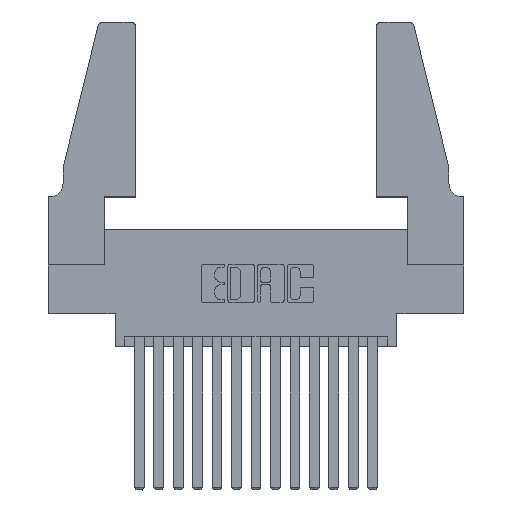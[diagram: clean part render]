
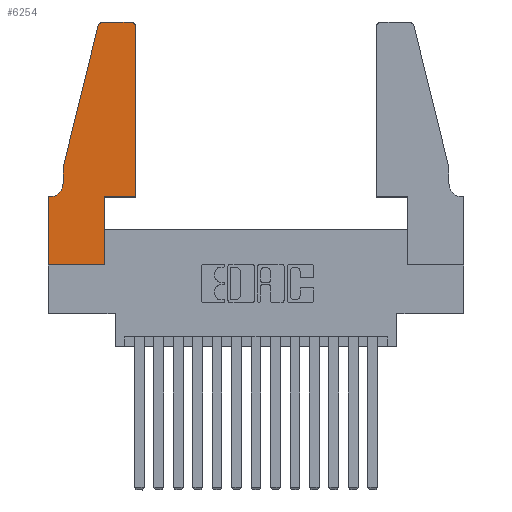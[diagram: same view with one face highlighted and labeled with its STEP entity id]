
A CAD part, top view. The second image highlights one B-rep face of the part: STEP entity #6254.
In plain terms, the highlighted planar face has unit normal (0, 0, 1).
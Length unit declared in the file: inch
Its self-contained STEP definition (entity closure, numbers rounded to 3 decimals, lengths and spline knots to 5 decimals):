
#33 = VERTEX_POINT ( 'NONE', #5022 ) ;
#185 = VECTOR ( 'NONE', #2375, 39.37008 ) ;
#260 = CARTESIAN_POINT ( 'NONE',  ( 0.2605, 1.25, 0.37 ) ) ;
#501 = DIRECTION ( 'NONE',  ( -0.239, -0.971, 0. ) ) ;
#542 = VERTEX_POINT ( 'NONE', #3157 ) ;
#551 = CARTESIAN_POINT ( 'NONE',  ( 0.0055, 0.35, 0.37 ) ) ;
#555 = CARTESIAN_POINT ( 'NONE',  ( 0., 0., 0.37 ) ) ;
#728 = EDGE_LOOP ( 'NONE', ( #1157, #2343, #8900, #1008, #6773, #13851, #2704, #11335, #4431, #1847, #6000, #14599 ) ) ;
#1008 = ORIENTED_EDGE ( 'NONE', *, *, #10303, .T. ) ;
#1157 = ORIENTED_EDGE ( 'NONE', *, *, #7819, .T. ) ;
#1281 = LINE ( 'NONE', #8338, #14203 ) ;
#1460 = EDGE_CURVE ( 'NONE', #542, #1535, #15334, .T. ) ;
#1535 = VERTEX_POINT ( 'NONE', #551 ) ;
#1579 = LINE ( 'NONE', #5400, #8222 ) ;
#1707 = AXIS2_PLACEMENT_3D ( 'NONE', #11863, #11811, #13019 ) ;
#1847 = ORIENTED_EDGE ( 'NONE', *, *, #3144, .T. ) ;
#2343 = ORIENTED_EDGE ( 'NONE', *, *, #10729, .T. ) ;
#2375 = DIRECTION ( 'NONE',  ( 1., 0., 0. ) ) ;
#2704 = ORIENTED_EDGE ( 'NONE', *, *, #3791, .T. ) ;
#2782 = LINE ( 'NONE', #3411, #4907 ) ;
#3086 = CARTESIAN_POINT ( 'NONE',  ( 0.4205, 1.25, 0.37 ) ) ;
#3144 = EDGE_CURVE ( 'NONE', #33, #7969, #6995, .T. ) ;
#3157 = CARTESIAN_POINT ( 'NONE',  ( 0.0755, 0.42, 0.37 ) ) ;
#3323 = CARTESIAN_POINT ( 'NONE',  ( 0.2865, 0.35, 0.37 ) ) ;
#3411 = CARTESIAN_POINT ( 'NONE',  ( 0., 0., 0.37 ) ) ;
#3791 = EDGE_CURVE ( 'NONE', #4390, #13098, #8411, .T. ) ;
#4056 = VERTEX_POINT ( 'NONE', #7187 ) ;
#4128 = CARTESIAN_POINT ( 'NONE',  ( 0.25487, 1.22718, 0.37 ) ) ;
#4390 = VERTEX_POINT ( 'NONE', #10632 ) ;
#4431 = ORIENTED_EDGE ( 'NONE', *, *, #7529, .T. ) ;
#4833 = PLANE ( 'NONE',  #11799 ) ;
#4902 = CARTESIAN_POINT ( 'NONE',  ( 0.0755, 0.5, 0.37 ) ) ;
#4907 = VECTOR ( 'NONE', #7054, 39.37008 ) ;
#5022 = CARTESIAN_POINT ( 'NONE',  ( 0.2865, 0.35, 0.37 ) ) ;
#5391 = CIRCLE ( 'NONE', #9222, 0.03 ) ;
#5400 = CARTESIAN_POINT ( 'NONE',  ( 0.0755, 0.5, 0.37 ) ) ;
#5651 = FACE_OUTER_BOUND ( 'NONE', #728, .T. ) ;
#5912 = CARTESIAN_POINT ( 'NONE',  ( 0., 0.35, 0.37 ) ) ;
#6000 = ORIENTED_EDGE ( 'NONE', *, *, #7105, .T. ) ;
#6004 = LINE ( 'NONE', #260, #13074 ) ;
#6099 = DIRECTION ( 'NONE',  ( 0., -1., 0. ) ) ;
#6254 = ADVANCED_FACE ( 'NONE', ( #5651 ), #4833, .T. ) ;
#6327 = EDGE_CURVE ( 'NONE', #6686, #4056, #1579, .T. ) ;
#6333 = CARTESIAN_POINT ( 'NONE',  ( 0.4505, 0.35, 0.37 ) ) ;
#6405 = LINE ( 'NONE', #11149, #8392 ) ;
#6648 = DIRECTION ( 'NONE',  ( 0., -1., 0. ) ) ;
#6686 = VERTEX_POINT ( 'NONE', #4128 ) ;
#6773 = ORIENTED_EDGE ( 'NONE', *, *, #1460, .T. ) ;
#6995 = LINE ( 'NONE', #6333, #185 ) ;
#7054 = DIRECTION ( 'NONE',  ( 1., 0., 0. ) ) ;
#7105 = EDGE_CURVE ( 'NONE', #7969, #13736, #6405, .T. ) ;
#7187 = CARTESIAN_POINT ( 'NONE',  ( 0.0755, 0.5, 0.37 ) ) ;
#7302 = LINE ( 'NONE', #4902, #13593 ) ;
#7529 = EDGE_CURVE ( 'NONE', #13959, #33, #9547, .T. ) ;
#7819 = EDGE_CURVE ( 'NONE', #12432, #11393, #6004, .T. ) ;
#7849 = CARTESIAN_POINT ( 'NONE',  ( 0., 0., 0.37 ) ) ;
#7969 = VERTEX_POINT ( 'NONE', #10036 ) ;
#8222 = VECTOR ( 'NONE', #501, 39.37008 ) ;
#8338 = CARTESIAN_POINT ( 'NONE',  ( 0.0755, 0.35, 0.37 ) ) ;
#8392 = VECTOR ( 'NONE', #13755, 39.37008 ) ;
#8411 = LINE ( 'NONE', #555, #10169 ) ;
#8900 = ORIENTED_EDGE ( 'NONE', *, *, #6327, .T. ) ;
#9218 = CARTESIAN_POINT ( 'NONE',  ( 0.2865, 0., 0.37 ) ) ;
#9222 = AXIS2_PLACEMENT_3D ( 'NONE', #14486, #9492, #10856 ) ;
#9356 = DIRECTION ( 'NONE',  ( 0., 1., 0. ) ) ;
#9492 = DIRECTION ( 'NONE',  ( 0., 0., 1. ) ) ;
#9547 = LINE ( 'NONE', #3323, #14077 ) ;
#9579 = CARTESIAN_POINT ( 'NONE',  ( 0.284, 1.25, 0.37 ) ) ;
#9611 = DIRECTION ( 'NONE',  ( 1., 0., 0. ) ) ;
#10036 = CARTESIAN_POINT ( 'NONE',  ( 0.4505, 0.35, 0.37 ) ) ;
#10044 = EDGE_CURVE ( 'NONE', #13736, #12432, #13369, .T. ) ;
#10169 = VECTOR ( 'NONE', #6648, 39.37008 ) ;
#10303 = EDGE_CURVE ( 'NONE', #4056, #542, #7302, .T. ) ;
#10632 = CARTESIAN_POINT ( 'NONE',  ( 0., 0.35, 0.37 ) ) ;
#10729 = EDGE_CURVE ( 'NONE', #11393, #6686, #5391, .T. ) ;
#10856 = DIRECTION ( 'NONE',  ( 1., 0., 0. ) ) ;
#11069 = DIRECTION ( 'NONE',  ( 0., 0., 1. ) ) ;
#11149 = CARTESIAN_POINT ( 'NONE',  ( 0.4505, 0.35, 0.37 ) ) ;
#11335 = ORIENTED_EDGE ( 'NONE', *, *, #14444, .T. ) ;
#11393 = VERTEX_POINT ( 'NONE', #9579 ) ;
#11504 = DIRECTION ( 'NONE',  ( -1., 0., 0. ) ) ;
#11799 = AXIS2_PLACEMENT_3D ( 'NONE', #5912, #11069, #13615 ) ;
#11811 = DIRECTION ( 'NONE',  ( 0., 0., -1. ) ) ;
#11863 = CARTESIAN_POINT ( 'NONE',  ( 0.0055, 0.42, 0.37 ) ) ;
#11930 = CARTESIAN_POINT ( 'NONE',  ( 0.4205, 1.22, 0.37 ) ) ;
#12118 = EDGE_CURVE ( 'NONE', #1535, #4390, #1281, .T. ) ;
#12432 = VERTEX_POINT ( 'NONE', #3086 ) ;
#12589 = AXIS2_PLACEMENT_3D ( 'NONE', #11930, #15740, #9611 ) ;
#13019 = DIRECTION ( 'NONE',  ( -1., 0., 0. ) ) ;
#13074 = VECTOR ( 'NONE', #11504, 39.37008 ) ;
#13098 = VERTEX_POINT ( 'NONE', #7849 ) ;
#13260 = DIRECTION ( 'NONE',  ( -1., 0., 0. ) ) ;
#13369 = CIRCLE ( 'NONE', #12589, 0.03 ) ;
#13593 = VECTOR ( 'NONE', #6099, 39.37008 ) ;
#13615 = DIRECTION ( 'NONE',  ( 1., 0., 0. ) ) ;
#13736 = VERTEX_POINT ( 'NONE', #15652 ) ;
#13755 = DIRECTION ( 'NONE',  ( 0., 1., 0. ) ) ;
#13851 = ORIENTED_EDGE ( 'NONE', *, *, #12118, .T. ) ;
#13959 = VERTEX_POINT ( 'NONE', #9218 ) ;
#14077 = VECTOR ( 'NONE', #9356, 39.37008 ) ;
#14203 = VECTOR ( 'NONE', #13260, 39.37008 ) ;
#14444 = EDGE_CURVE ( 'NONE', #13098, #13959, #2782, .T. ) ;
#14486 = CARTESIAN_POINT ( 'NONE',  ( 0.284, 1.22, 0.37 ) ) ;
#14599 = ORIENTED_EDGE ( 'NONE', *, *, #10044, .T. ) ;
#15334 = CIRCLE ( 'NONE', #1707, 0.07 ) ;
#15652 = CARTESIAN_POINT ( 'NONE',  ( 0.4505, 1.22, 0.37 ) ) ;
#15740 = DIRECTION ( 'NONE',  ( 0., 0., 1. ) ) ;
